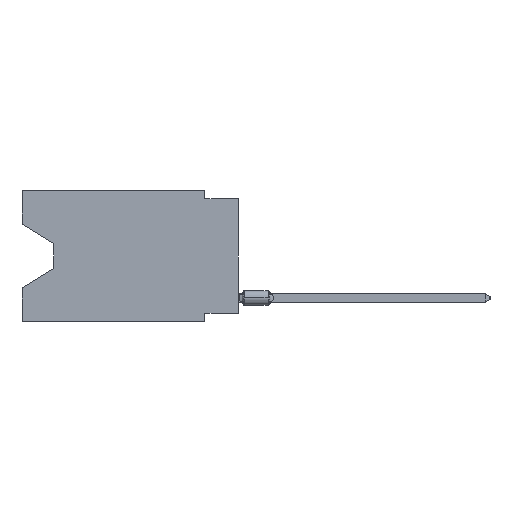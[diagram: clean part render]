
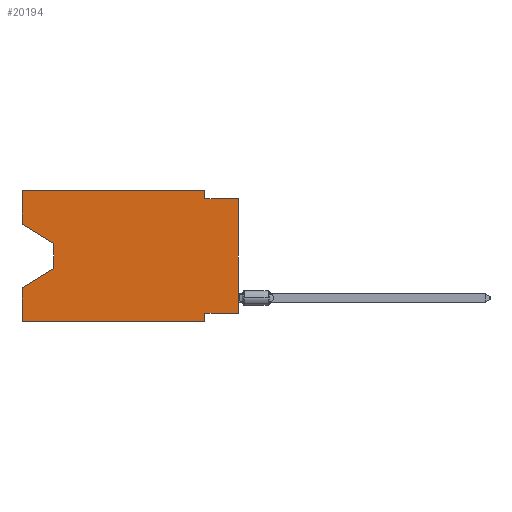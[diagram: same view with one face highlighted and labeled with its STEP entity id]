
A CAD part, left-side view. The second image highlights one B-rep face of the part: STEP entity #20194.
In plain terms, the highlighted planar face has unit normal (-1, 0, 0).
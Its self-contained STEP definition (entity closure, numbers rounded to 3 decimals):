
#277 = VECTOR ( 'NONE', #30390, 1000. ) ;
#1390 = ORIENTED_EDGE ( 'NONE', *, *, #37626, .F. ) ;
#3379 = CARTESIAN_POINT ( 'NONE',  ( 0., 13.97, -5.893 ) ) ;
#3895 = ORIENTED_EDGE ( 'NONE', *, *, #21455, .T. ) ;
#3996 = DIRECTION ( 'NONE',  ( 0., 0., -1. ) ) ;
#4159 = VERTEX_POINT ( 'NONE', #59339 ) ;
#5481 = CARTESIAN_POINT ( 'NONE',  ( 0., 2.54, -9.906 ) ) ;
#6262 = ORIENTED_EDGE ( 'NONE', *, *, #69576, .F. ) ;
#8344 = DIRECTION ( 'NONE',  ( 1., 0., 0. ) ) ;
#8578 = VECTOR ( 'NONE', #19771, 1000. ) ;
#8714 = LINE ( 'NONE', #30833, #69342 ) ;
#9668 = VERTEX_POINT ( 'NONE', #31840 ) ;
#10142 = DIRECTION ( 'NONE',  ( 0., 0., 1. ) ) ;
#11092 = ORIENTED_EDGE ( 'NONE', *, *, #37921, .T. ) ;
#11392 = VECTOR ( 'NONE', #60356, 1000. ) ;
#11955 = EDGE_CURVE ( 'NONE', #52207, #60780, #25210, .T. ) ;
#14170 = VERTEX_POINT ( 'NONE', #71409 ) ;
#14482 = ORIENTED_EDGE ( 'NONE', *, *, #62546, .T. ) ;
#14662 = ORIENTED_EDGE ( 'NONE', *, *, #69775, .T. ) ;
#14868 = LINE ( 'NONE', #43509, #42413 ) ;
#15056 = EDGE_CURVE ( 'NONE', #69315, #19025, #14868, .T. ) ;
#15148 = CARTESIAN_POINT ( 'NONE',  ( 0., 16.383, -7.36 ) ) ;
#16194 = CARTESIAN_POINT ( 'NONE',  ( 0., 0., -9.271 ) ) ;
#16621 = DIRECTION ( 'NONE',  ( 0., 0., 1. ) ) ;
#17004 = LINE ( 'NONE', #38780, #26856 ) ;
#18857 = DIRECTION ( 'NONE',  ( 0., -1., 0. ) ) ;
#18897 = CARTESIAN_POINT ( 'NONE',  ( 0., 0., -0.635 ) ) ;
#19025 = VERTEX_POINT ( 'NONE', #47792 ) ;
#19771 = DIRECTION ( 'NONE',  ( 0., 0., -1. ) ) ;
#19933 = EDGE_CURVE ( 'NONE', #60257, #46122, #28309, .T. ) ;
#20146 = VECTOR ( 'NONE', #16621, 1000. ) ;
#20194 = ADVANCED_FACE ( 'NONE', ( #70698 ), #58032, .F. ) ;
#21106 = VECTOR ( 'NONE', #66039, 1000. ) ;
#21455 = EDGE_CURVE ( 'NONE', #4159, #52207, #8714, .T. ) ;
#22028 = CARTESIAN_POINT ( 'NONE',  ( 0., 16.383, 0. ) ) ;
#23183 = CARTESIAN_POINT ( 'NONE',  ( 0., 16.383, -9.906 ) ) ;
#23772 = CARTESIAN_POINT ( 'NONE',  ( 0., 13.97, -4.013 ) ) ;
#25210 = LINE ( 'NONE', #23772, #8578 ) ;
#26856 = VECTOR ( 'NONE', #60899, 1000. ) ;
#28125 = VERTEX_POINT ( 'NONE', #23183 ) ;
#28309 = LINE ( 'NONE', #5481, #21106 ) ;
#28647 = CARTESIAN_POINT ( 'NONE',  ( 0., 0., -0.635 ) ) ;
#28840 = DIRECTION ( 'NONE',  ( 0., 1., 0. ) ) ;
#29689 = VERTEX_POINT ( 'NONE', #18897 ) ;
#30390 = DIRECTION ( 'NONE',  ( 0., -1., 0. ) ) ;
#30833 = CARTESIAN_POINT ( 'NONE',  ( 0., 16.383, -2.546 ) ) ;
#31840 = CARTESIAN_POINT ( 'NONE',  ( 0., 2.54, -0.635 ) ) ;
#32239 = DIRECTION ( 'NONE',  ( 0., -1., 0. ) ) ;
#33351 = VERTEX_POINT ( 'NONE', #15148 ) ;
#33479 = CARTESIAN_POINT ( 'NONE',  ( 0., 13.97, -5.893 ) ) ;
#33786 = VECTOR ( 'NONE', #18857, 1000. ) ;
#34276 = ORIENTED_EDGE ( 'NONE', *, *, #49211, .F. ) ;
#37626 = EDGE_CURVE ( 'NONE', #14170, #60257, #65861, .T. ) ;
#37718 = LINE ( 'NONE', #70021, #61398 ) ;
#37921 = EDGE_CURVE ( 'NONE', #60780, #33351, #49834, .T. ) ;
#38197 = CARTESIAN_POINT ( 'NONE',  ( 0., 2.54, 0. ) ) ;
#38780 = CARTESIAN_POINT ( 'NONE',  ( 0., 16.383, 0. ) ) ;
#39445 = ORIENTED_EDGE ( 'NONE', *, *, #45959, .F. ) ;
#41399 = ORIENTED_EDGE ( 'NONE', *, *, #15056, .F. ) ;
#42413 = VECTOR ( 'NONE', #32239, 1000. ) ;
#43442 = VECTOR ( 'NONE', #48031, 1000. ) ;
#43509 = CARTESIAN_POINT ( 'NONE',  ( 0., 16.383, 0. ) ) ;
#43863 = VECTOR ( 'NONE', #28840, 1000. ) ;
#44168 = LINE ( 'NONE', #22028, #20146 ) ;
#45151 = CARTESIAN_POINT ( 'NONE',  ( 0., 13.97, -4.013 ) ) ;
#45703 = EDGE_LOOP ( 'NONE', ( #3895, #48085, #11092, #39445, #14662, #57693, #1390, #14482, #53381, #34276, #41399, #6262 ) ) ;
#45959 = EDGE_CURVE ( 'NONE', #28125, #33351, #44168, .T. ) ;
#46122 = VERTEX_POINT ( 'NONE', #64065 ) ;
#47071 = CARTESIAN_POINT ( 'NONE',  ( 0., 16.383, -9.906 ) ) ;
#47792 = CARTESIAN_POINT ( 'NONE',  ( 0., 2.54, 0. ) ) ;
#48031 = DIRECTION ( 'NONE',  ( 0., 0., -1. ) ) ;
#48085 = ORIENTED_EDGE ( 'NONE', *, *, #11955, .T. ) ;
#49211 = EDGE_CURVE ( 'NONE', #19025, #9668, #60693, .T. ) ;
#49834 = LINE ( 'NONE', #33479, #11392 ) ;
#50788 = LINE ( 'NONE', #28647, #33786 ) ;
#52050 = CARTESIAN_POINT ( 'NONE',  ( 0., 2.54, -9.271 ) ) ;
#52207 = VERTEX_POINT ( 'NONE', #45151 ) ;
#53224 = LINE ( 'NONE', #47071, #277 ) ;
#53381 = ORIENTED_EDGE ( 'NONE', *, *, #69207, .F. ) ;
#53671 = CARTESIAN_POINT ( 'NONE',  ( 0., 16.383, 0. ) ) ;
#57693 = ORIENTED_EDGE ( 'NONE', *, *, #19933, .F. ) ;
#58032 = PLANE ( 'NONE',  #67451 ) ;
#58753 = CARTESIAN_POINT ( 'NONE',  ( 0., 16.383, 0. ) ) ;
#59339 = CARTESIAN_POINT ( 'NONE',  ( 0., 16.383, -2.546 ) ) ;
#60257 = VERTEX_POINT ( 'NONE', #52050 ) ;
#60342 = DIRECTION ( 'NONE',  ( 0., -0.855, -0.519 ) ) ;
#60356 = DIRECTION ( 'NONE',  ( 0., 0.855, -0.519 ) ) ;
#60693 = LINE ( 'NONE', #38197, #43442 ) ;
#60780 = VERTEX_POINT ( 'NONE', #3379 ) ;
#60899 = DIRECTION ( 'NONE',  ( 0., 0., 1. ) ) ;
#61398 = VECTOR ( 'NONE', #10142, 1000. ) ;
#62546 = EDGE_CURVE ( 'NONE', #14170, #29689, #37718, .T. ) ;
#64065 = CARTESIAN_POINT ( 'NONE',  ( 0., 2.54, -9.906 ) ) ;
#65861 = LINE ( 'NONE', #16194, #43863 ) ;
#66039 = DIRECTION ( 'NONE',  ( 0., 0., -1. ) ) ;
#67451 = AXIS2_PLACEMENT_3D ( 'NONE', #53671, #8344, #3996 ) ;
#69207 = EDGE_CURVE ( 'NONE', #9668, #29689, #50788, .T. ) ;
#69315 = VERTEX_POINT ( 'NONE', #58753 ) ;
#69342 = VECTOR ( 'NONE', #60342, 1000. ) ;
#69576 = EDGE_CURVE ( 'NONE', #4159, #69315, #17004, .T. ) ;
#69775 = EDGE_CURVE ( 'NONE', #28125, #46122, #53224, .T. ) ;
#70021 = CARTESIAN_POINT ( 'NONE',  ( 0., 0., 0. ) ) ;
#70698 = FACE_OUTER_BOUND ( 'NONE', #45703, .T. ) ;
#71409 = CARTESIAN_POINT ( 'NONE',  ( 0., 0., -9.271 ) ) ;
